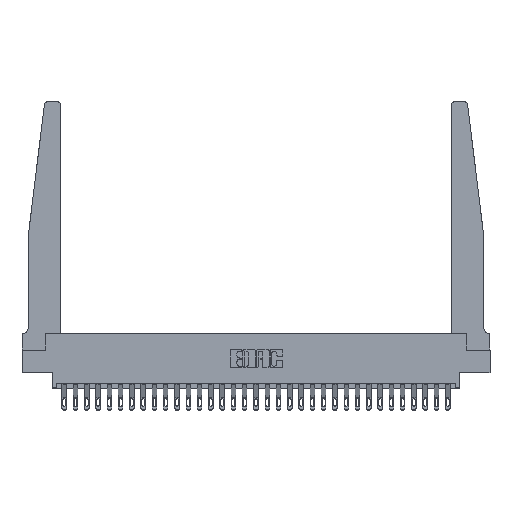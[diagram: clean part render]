
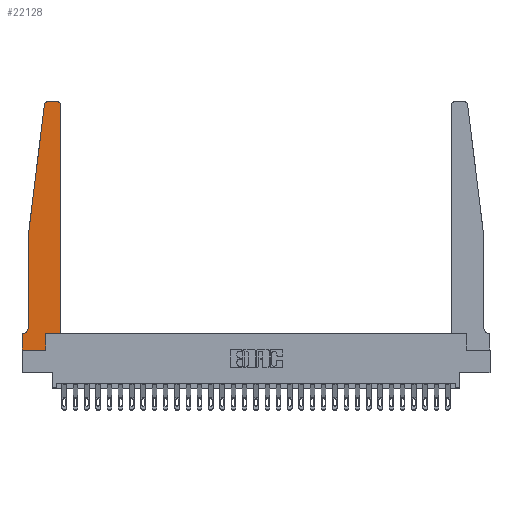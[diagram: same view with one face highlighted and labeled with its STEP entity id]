
A CAD part, top view. The second image highlights one B-rep face of the part: STEP entity #22128.
In plain terms, the highlighted planar face has unit normal (0, 0, 1).
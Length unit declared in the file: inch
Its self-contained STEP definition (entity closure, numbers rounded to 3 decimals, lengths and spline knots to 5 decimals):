
#168 = CARTESIAN_POINT ( 'NONE',  ( 0., 0., 0.37 ) ) ;
#694 = EDGE_CURVE ( 'NONE', #1529, #8893, #10132, .T. ) ;
#1170 = CARTESIAN_POINT ( 'NONE',  ( 0.27653, 2.72, 0.37 ) ) ;
#1378 = ORIENTED_EDGE ( 'NONE', *, *, #5876, .T. ) ;
#1389 = DIRECTION ( 'NONE',  ( 0., -1., 0. ) ) ;
#1505 = VERTEX_POINT ( 'NONE', #12387 ) ;
#1529 = VERTEX_POINT ( 'NONE', #28818 ) ;
#2519 = CARTESIAN_POINT ( 'NONE',  ( 0.065, 1.25, 0.37 ) ) ;
#3103 = DIRECTION ( 'NONE',  ( 0., 0., 1. ) ) ;
#3125 = CARTESIAN_POINT ( 'NONE',  ( 0.065, 0.1875, 0.37 ) ) ;
#3331 = ORIENTED_EDGE ( 'NONE', *, *, #8817, .T. ) ;
#3479 = CIRCLE ( 'NONE', #25864, 0.03 ) ;
#3677 = VECTOR ( 'NONE', #1389, 39.37008 ) ;
#3918 = CARTESIAN_POINT ( 'NONE',  ( 0.065, 1.25, 0.37 ) ) ;
#4258 = CARTESIAN_POINT ( 'NONE',  ( 0.2605, 0., 0.37 ) ) ;
#4415 = AXIS2_PLACEMENT_3D ( 'NONE', #24612, #26419, #19701 ) ;
#4572 = DIRECTION ( 'NONE',  ( 1., 0., 0. ) ) ;
#5062 = VERTEX_POINT ( 'NONE', #19791 ) ;
#5366 = EDGE_CURVE ( 'NONE', #9994, #5062, #7834, .T. ) ;
#5726 = DIRECTION ( 'NONE',  ( 0., -1., 0. ) ) ;
#5876 = EDGE_CURVE ( 'NONE', #8893, #6996, #27278, .T. ) ;
#5907 = DIRECTION ( 'NONE',  ( 1., 0., 0. ) ) ;
#6028 = CARTESIAN_POINT ( 'NONE',  ( 0.065, 1.25, 0.37 ) ) ;
#6453 = VERTEX_POINT ( 'NONE', #13658 ) ;
#6996 = VERTEX_POINT ( 'NONE', #26145 ) ;
#7149 = VECTOR ( 'NONE', #4572, 39.37008 ) ;
#7164 = LINE ( 'NONE', #16110, #16388 ) ;
#7573 = DIRECTION ( 'NONE',  ( 1., 0., 0. ) ) ;
#7649 = ORIENTED_EDGE ( 'NONE', *, *, #20426, .T. ) ;
#7834 = LINE ( 'NONE', #25727, #13171 ) ;
#8817 = EDGE_CURVE ( 'NONE', #24075, #21128, #15251, .T. ) ;
#8893 = VERTEX_POINT ( 'NONE', #18071 ) ;
#9371 = DIRECTION ( 'NONE',  ( -0.122, -0.992, 0. ) ) ;
#9488 = CIRCLE ( 'NONE', #26166, 0.05 ) ;
#9699 = DIRECTION ( 'NONE',  ( 1., 0., 0. ) ) ;
#9788 = VECTOR ( 'NONE', #13783, 39.37008 ) ;
#9846 = DIRECTION ( 'NONE',  ( -1., 0., 0. ) ) ;
#9994 = VERTEX_POINT ( 'NONE', #27853 ) ;
#10132 = LINE ( 'NONE', #3125, #22303 ) ;
#10180 = VERTEX_POINT ( 'NONE', #29140 ) ;
#10328 = ORIENTED_EDGE ( 'NONE', *, *, #17824, .T. ) ;
#11677 = ORIENTED_EDGE ( 'NONE', *, *, #15147, .T. ) ;
#11731 = CARTESIAN_POINT ( 'NONE',  ( 0.015, 0.2375, 0.37 ) ) ;
#11868 = DIRECTION ( 'NONE',  ( -1., 0., 0. ) ) ;
#12238 = ORIENTED_EDGE ( 'NONE', *, *, #5366, .T. ) ;
#12387 = CARTESIAN_POINT ( 'NONE',  ( 0.2605, 0.18, 0.37 ) ) ;
#12896 = FACE_OUTER_BOUND ( 'NONE', #15013, .T. ) ;
#13171 = VECTOR ( 'NONE', #16918, 39.37008 ) ;
#13658 = CARTESIAN_POINT ( 'NONE',  ( 0.27653, 2.75, 0.37 ) ) ;
#13783 = DIRECTION ( 'NONE',  ( 0., 1., 0. ) ) ;
#14310 = LINE ( 'NONE', #168, #27826 ) ;
#14991 = PLANE ( 'NONE',  #28643 ) ;
#15013 = EDGE_LOOP ( 'NONE', ( #21265, #22751, #26467, #3331, #10328, #22617, #1378, #26430, #21871, #7649, #12238, #11677 ) ) ;
#15147 = EDGE_CURVE ( 'NONE', #5062, #16533, #17272, .T. ) ;
#15251 = LINE ( 'NONE', #6028, #18055 ) ;
#16110 = CARTESIAN_POINT ( 'NONE',  ( 0.25, 2.75, 0.37 ) ) ;
#16388 = VECTOR ( 'NONE', #9846, 39.37008 ) ;
#16533 = VERTEX_POINT ( 'NONE', #20363 ) ;
#16683 = DIRECTION ( 'NONE',  ( -1., 0., 0. ) ) ;
#16918 = DIRECTION ( 'NONE',  ( 0., 1., 0. ) ) ;
#17272 = CIRCLE ( 'NONE', #4415, 0.03 ) ;
#17761 = CARTESIAN_POINT ( 'NONE',  ( 0.425, 0.18, 0.37 ) ) ;
#17824 = EDGE_CURVE ( 'NONE', #21128, #1529, #9488, .T. ) ;
#18024 = CARTESIAN_POINT ( 'NONE',  ( 0., 0., 0.37 ) ) ;
#18055 = VECTOR ( 'NONE', #5726, 39.37008 ) ;
#18071 = CARTESIAN_POINT ( 'NONE',  ( 0., 0.1875, 0.37 ) ) ;
#18318 = LINE ( 'NONE', #2519, #24503 ) ;
#19701 = DIRECTION ( 'NONE',  ( 1., 0., 0. ) ) ;
#19791 = CARTESIAN_POINT ( 'NONE',  ( 0.425, 2.72, 0.37 ) ) ;
#20363 = CARTESIAN_POINT ( 'NONE',  ( 0.395, 2.75, 0.37 ) ) ;
#20426 = EDGE_CURVE ( 'NONE', #1505, #9994, #24996, .T. ) ;
#21128 = VERTEX_POINT ( 'NONE', #22066 ) ;
#21265 = ORIENTED_EDGE ( 'NONE', *, *, #25498, .T. ) ;
#21847 = DIRECTION ( 'NONE',  ( 0., 0., 1. ) ) ;
#21871 = ORIENTED_EDGE ( 'NONE', *, *, #28862, .T. ) ;
#22066 = CARTESIAN_POINT ( 'NONE',  ( 0.065, 0.2375, 0.37 ) ) ;
#22128 = ADVANCED_FACE ( 'NONE', ( #12896 ), #14991, .T. ) ;
#22238 = VERTEX_POINT ( 'NONE', #4258 ) ;
#22303 = VECTOR ( 'NONE', #16683, 39.37008 ) ;
#22617 = ORIENTED_EDGE ( 'NONE', *, *, #694, .T. ) ;
#22751 = ORIENTED_EDGE ( 'NONE', *, *, #26045, .T. ) ;
#22905 = DIRECTION ( 'NONE',  ( 0., 0., -1. ) ) ;
#24075 = VERTEX_POINT ( 'NONE', #3918 ) ;
#24503 = VECTOR ( 'NONE', #9371, 39.37008 ) ;
#24612 = CARTESIAN_POINT ( 'NONE',  ( 0.395, 2.72, 0.37 ) ) ;
#24982 = LINE ( 'NONE', #25128, #9788 ) ;
#24996 = LINE ( 'NONE', #17761, #7149 ) ;
#25128 = CARTESIAN_POINT ( 'NONE',  ( 0.2605, 0.18, 0.37 ) ) ;
#25498 = EDGE_CURVE ( 'NONE', #16533, #6453, #7164, .T. ) ;
#25536 = EDGE_CURVE ( 'NONE', #6996, #22238, #14310, .T. ) ;
#25727 = CARTESIAN_POINT ( 'NONE',  ( 0.425, 0.18, 0.37 ) ) ;
#25864 = AXIS2_PLACEMENT_3D ( 'NONE', #1170, #3103, #7573 ) ;
#26045 = EDGE_CURVE ( 'NONE', #6453, #10180, #3479, .T. ) ;
#26145 = CARTESIAN_POINT ( 'NONE',  ( 0., 0., 0.37 ) ) ;
#26166 = AXIS2_PLACEMENT_3D ( 'NONE', #11731, #22905, #11868 ) ;
#26337 = CARTESIAN_POINT ( 'NONE',  ( 0., 0.1875, 0.37 ) ) ;
#26419 = DIRECTION ( 'NONE',  ( 0., 0., 1. ) ) ;
#26430 = ORIENTED_EDGE ( 'NONE', *, *, #25536, .T. ) ;
#26467 = ORIENTED_EDGE ( 'NONE', *, *, #27213, .T. ) ;
#27213 = EDGE_CURVE ( 'NONE', #10180, #24075, #18318, .T. ) ;
#27278 = LINE ( 'NONE', #18024, #3677 ) ;
#27826 = VECTOR ( 'NONE', #9699, 39.37008 ) ;
#27853 = CARTESIAN_POINT ( 'NONE',  ( 0.425, 0.18, 0.37 ) ) ;
#28643 = AXIS2_PLACEMENT_3D ( 'NONE', #26337, #21847, #5907 ) ;
#28818 = CARTESIAN_POINT ( 'NONE',  ( 0.015, 0.1875, 0.37 ) ) ;
#28862 = EDGE_CURVE ( 'NONE', #22238, #1505, #24982, .T. ) ;
#29140 = CARTESIAN_POINT ( 'NONE',  ( 0.24675, 2.72367, 0.37 ) ) ;
